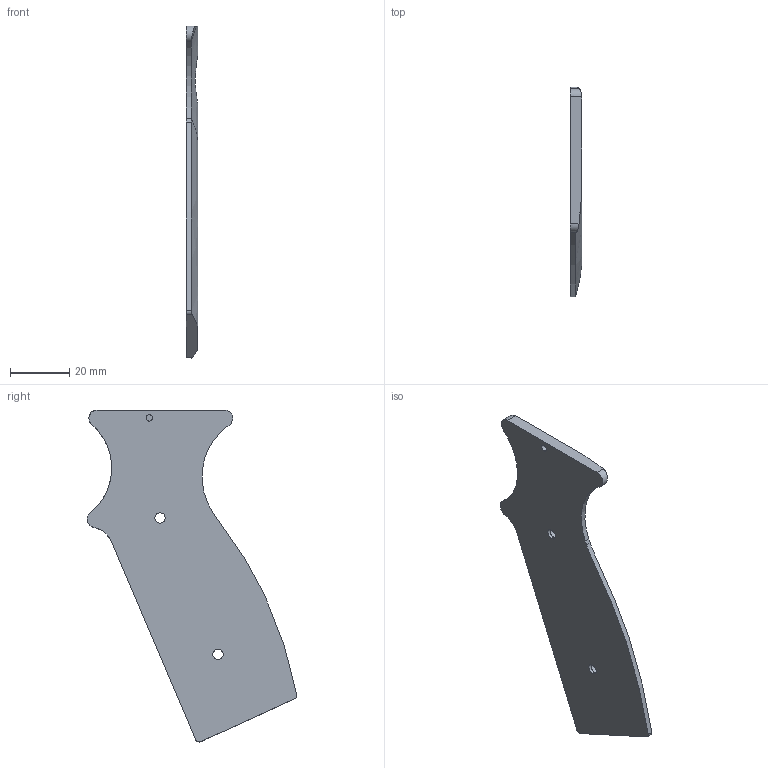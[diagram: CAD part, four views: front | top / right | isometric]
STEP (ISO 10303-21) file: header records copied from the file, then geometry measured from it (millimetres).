
FILE_DESCRIPTION (( 'STEP AP214' ), '1' );
FILE_NAME ('Grip_Thin_Basic_R_V10.STEP', '2025-07-07T03:51:16', ( '' ), ( '' ), 'SwSTEP 2.0', 'SolidWorks 2020', '' );
FILE_SCHEMA (( 'AUTOMOTIVE_DESIGN' ));
Length unit declared in the file: millimetre
Products named in the file (1): Grip_Thin_Basic_R_V10
Bounding box: 4 x 70.74 x 112.04 mm (x, y, z)
Volume: 14289.5 mm3; surface area: 9400.9 mm2
Topology: 1 solids, 1 shells, 40 faces, 99 edges, 64 vertices
Faces by surface type: cylinder 17, bspline 13, plane 10
Entity records: 1858 total; most frequent: CARTESIAN_POINT 947, ORIENTED_EDGE 198, DIRECTION 150, EDGE_CURVE 99, VERTEX_POINT 64, AXIS2_PLACEMENT_3D 58, EDGE_LOOP 47, FACE_OUTER_BOUND 40
